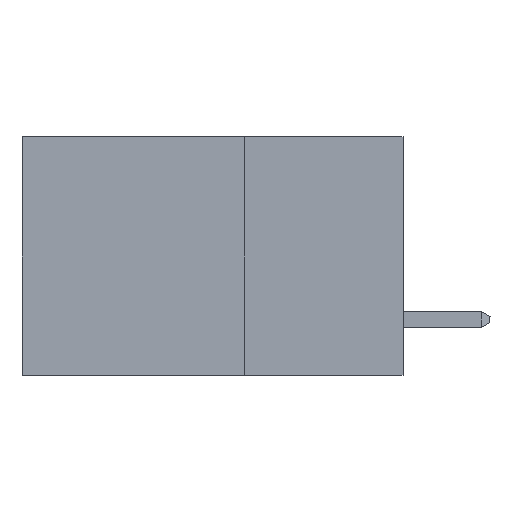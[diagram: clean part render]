
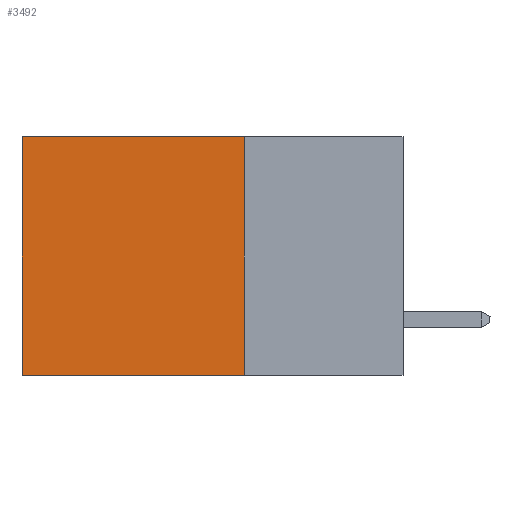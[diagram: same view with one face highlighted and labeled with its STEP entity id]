
A CAD part, left-side view. The second image highlights one B-rep face of the part: STEP entity #3492.
In plain terms, the highlighted planar face has unit normal (-1, 0, 0).
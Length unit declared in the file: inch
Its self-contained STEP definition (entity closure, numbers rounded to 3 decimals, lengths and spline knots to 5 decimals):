
#305 = LINE ( 'NONE', #3783, #12804 ) ;
#981 = DIRECTION ( 'NONE',  ( 0., 1., 0. ) ) ;
#1794 = VECTOR ( 'NONE', #981, 39.37008 ) ;
#2112 = DIRECTION ( 'NONE',  ( 1., 0., 0. ) ) ;
#2964 = EDGE_CURVE ( 'NONE', #10420, #13688, #9777, .T. ) ;
#2985 = CARTESIAN_POINT ( 'NONE',  ( 0.2875, 0.25, -0.375 ) ) ;
#3492 = ADVANCED_FACE ( 'NONE', ( #6622 ), #10103, .F. ) ;
#3783 = CARTESIAN_POINT ( 'NONE',  ( 0.2875, 0.25, -0.375 ) ) ;
#3919 = VERTEX_POINT ( 'NONE', #4213 ) ;
#4022 = CARTESIAN_POINT ( 'NONE',  ( 0.2875, 0.6, 0. ) ) ;
#4213 = CARTESIAN_POINT ( 'NONE',  ( 0.2875, 0.6, -0.375 ) ) ;
#4571 = AXIS2_PLACEMENT_3D ( 'NONE', #13249, #2112, #13385 ) ;
#4660 = DIRECTION ( 'NONE',  ( 0., 0., -1. ) ) ;
#5428 = VECTOR ( 'NONE', #11566, 39.37008 ) ;
#6105 = VECTOR ( 'NONE', #8784, 39.37008 ) ;
#6598 = EDGE_LOOP ( 'NONE', ( #13764, #10384, #13344, #11807 ) ) ;
#6622 = FACE_OUTER_BOUND ( 'NONE', #6598, .T. ) ;
#7129 = CARTESIAN_POINT ( 'NONE',  ( 0.2875, 0.6, -0.375 ) ) ;
#8712 = CARTESIAN_POINT ( 'NONE',  ( 0.2875, 0.25, -0.375 ) ) ;
#8784 = DIRECTION ( 'NONE',  ( 0., 1., 0. ) ) ;
#9450 = EDGE_CURVE ( 'NONE', #13688, #3919, #10480, .T. ) ;
#9777 = LINE ( 'NONE', #11889, #1794 ) ;
#10103 = PLANE ( 'NONE',  #4571 ) ;
#10384 = ORIENTED_EDGE ( 'NONE', *, *, #11366, .F. ) ;
#10420 = VERTEX_POINT ( 'NONE', #12470 ) ;
#10480 = LINE ( 'NONE', #7129, #5428 ) ;
#11366 = EDGE_CURVE ( 'NONE', #14046, #3919, #14298, .T. ) ;
#11566 = DIRECTION ( 'NONE',  ( 0., 0., -1. ) ) ;
#11807 = ORIENTED_EDGE ( 'NONE', *, *, #2964, .T. ) ;
#11889 = CARTESIAN_POINT ( 'NONE',  ( 0.2875, 0.25, 0. ) ) ;
#12470 = CARTESIAN_POINT ( 'NONE',  ( 0.2875, 0.25, 0. ) ) ;
#12804 = VECTOR ( 'NONE', #4660, 39.37008 ) ;
#13249 = CARTESIAN_POINT ( 'NONE',  ( 0.2875, 0.25, -0.375 ) ) ;
#13344 = ORIENTED_EDGE ( 'NONE', *, *, #13960, .F. ) ;
#13385 = DIRECTION ( 'NONE',  ( 0., 0., -1. ) ) ;
#13688 = VERTEX_POINT ( 'NONE', #4022 ) ;
#13764 = ORIENTED_EDGE ( 'NONE', *, *, #9450, .T. ) ;
#13960 = EDGE_CURVE ( 'NONE', #10420, #14046, #305, .T. ) ;
#14046 = VERTEX_POINT ( 'NONE', #2985 ) ;
#14298 = LINE ( 'NONE', #8712, #6105 ) ;
